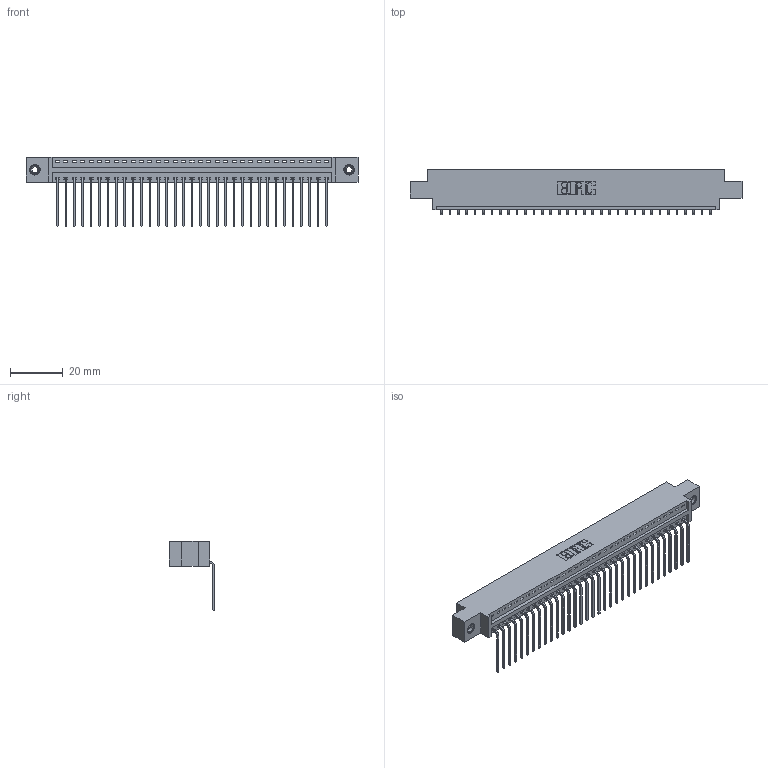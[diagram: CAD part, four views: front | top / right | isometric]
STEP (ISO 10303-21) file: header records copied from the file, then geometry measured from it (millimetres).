
FILE_DESCRIPTION (( 'STEP AP203' ), '1' );
FILE_NAME ('396-033-559-608.STEP', '2018-09-05T23:44:08', ( '' ), ( '' ), 'SwSTEP 2.0', 'SolidWorks 2016', '' );
FILE_SCHEMA (( 'CONFIG_CONTROL_DESIGN' ));
Length unit declared in the file: inch
Products named in the file (4): 345-292-001_558 559 Tail - 1; 345-250-001_345-250-003-102; 396-033-559-608; 346 Part_0.170 Offset - 0.156 Dia-TI
Assembly tree (36 placements, depth 2):
  396-033-559-608
    346 Part_0.170 Offset - 0.156 Dia-TI
    345-292-001_558 559 Tail - 1  x33
    345-250-001_345-250-003-102  x2
Bounding box: 125.35 x 17.08 x 26.16 mm (x, y, z)
Volume: 11885.5 mm3; surface area: 15596.3 mm2
Topology: 36 solids, 36 shells, 2166 faces, 6483 edges, 4270 vertices
Faces by surface type: plane 1498, cylinder 652, cone 12, torus 4
Entity records: 23094 total; most frequent: CARTESIAN_POINT 3946, ORIENTED_EDGE 3906, DIRECTION 3517, EDGE_CURVE 1953, VECTOR 1669, LINE 1669, VERTEX_POINT 1296, AXIS2_PLACEMENT_3D 924
